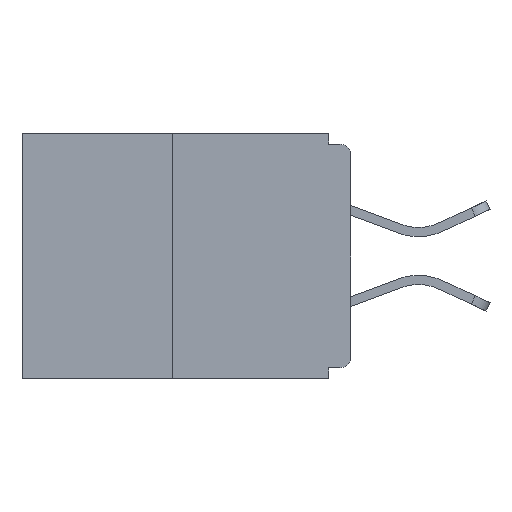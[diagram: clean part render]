
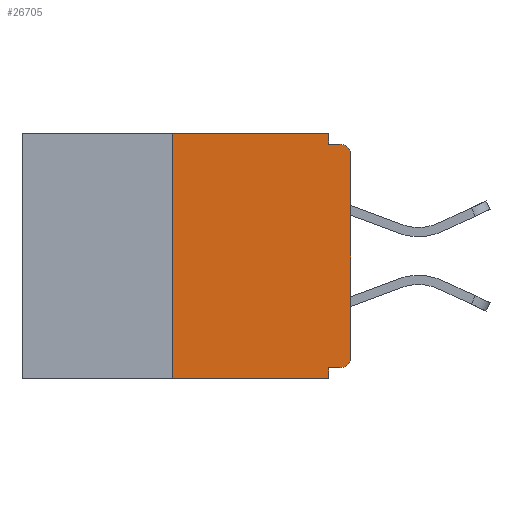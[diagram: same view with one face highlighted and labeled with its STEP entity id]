
A CAD part, left-side view. The second image highlights one B-rep face of the part: STEP entity #26705.
In plain terms, the highlighted planar face has unit normal (-1, 0, 0).
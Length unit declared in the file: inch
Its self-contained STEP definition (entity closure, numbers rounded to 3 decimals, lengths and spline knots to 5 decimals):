
#169 = VECTOR ( 'NONE', #17316, 39.37008 ) ;
#370 = ORIENTED_EDGE ( 'NONE', *, *, #10668, .T. ) ;
#379 = ORIENTED_EDGE ( 'NONE', *, *, #18137, .T. ) ;
#543 = DIRECTION ( 'NONE',  ( 0., 0., -1. ) ) ;
#657 = EDGE_LOOP ( 'NONE', ( #15188, #1661, #379, #4554, #2257, #5681, #370, #24033, #15216, #9652 ) ) ;
#1530 = DIRECTION ( 'NONE',  ( 0., 0., -1. ) ) ;
#1661 = ORIENTED_EDGE ( 'NONE', *, *, #25469, .F. ) ;
#1874 = VECTOR ( 'NONE', #26243, 39.37008 ) ;
#2257 = ORIENTED_EDGE ( 'NONE', *, *, #19185, .F. ) ;
#2644 = VECTOR ( 'NONE', #9814, 39.37008 ) ;
#2871 = VERTEX_POINT ( 'NONE', #27131 ) ;
#3639 = CARTESIAN_POINT ( 'NONE',  ( 0., 0.031, -0.328 ) ) ;
#3929 = VECTOR ( 'NONE', #16090, 39.37008 ) ;
#4485 = VERTEX_POINT ( 'NONE', #14809 ) ;
#4554 = ORIENTED_EDGE ( 'NONE', *, *, #28223, .F. ) ;
#4735 = DIRECTION ( 'NONE',  ( 0., 0., 1. ) ) ;
#5041 = EDGE_CURVE ( 'NONE', #23980, #18617, #19568, .T. ) ;
#5166 = AXIS2_PLACEMENT_3D ( 'NONE', #13131, #8432, #1530 ) ;
#5470 = LINE ( 'NONE', #19295, #26489 ) ;
#5681 = ORIENTED_EDGE ( 'NONE', *, *, #7123, .T. ) ;
#6280 = CARTESIAN_POINT ( 'NONE',  ( 0., 0.25, -0.343 ) ) ;
#7097 = CARTESIAN_POINT ( 'NONE',  ( 0., 0.25, 0. ) ) ;
#7123 = EDGE_CURVE ( 'NONE', #8736, #4485, #11064, .T. ) ;
#7246 = CARTESIAN_POINT ( 'NONE',  ( 0., 0.46, 0. ) ) ;
#7988 = LINE ( 'NONE', #18563, #3929 ) ;
#8432 = DIRECTION ( 'NONE',  ( -1., 0., 0. ) ) ;
#8517 = AXIS2_PLACEMENT_3D ( 'NONE', #17301, #24214, #19564 ) ;
#8670 = VERTEX_POINT ( 'NONE', #29027 ) ;
#8736 = VERTEX_POINT ( 'NONE', #10811 ) ;
#9028 = LINE ( 'NONE', #7097, #27049 ) ;
#9652 = ORIENTED_EDGE ( 'NONE', *, *, #22986, .F. ) ;
#9814 = DIRECTION ( 'NONE',  ( 0., -1., 0. ) ) ;
#10073 = VERTEX_POINT ( 'NONE', #18894 ) ;
#10401 = CARTESIAN_POINT ( 'NONE',  ( 0., 0., -0.328 ) ) ;
#10576 = DIRECTION ( 'NONE',  ( 0., 0., -1. ) ) ;
#10668 = EDGE_CURVE ( 'NONE', #4485, #8670, #15985, .T. ) ;
#10811 = CARTESIAN_POINT ( 'NONE',  ( 0., 0.015, -0.328 ) ) ;
#11064 = CIRCLE ( 'NONE', #8517, 0.015 ) ;
#11095 = LINE ( 'NONE', #23875, #1874 ) ;
#11470 = VERTEX_POINT ( 'NONE', #20252 ) ;
#13026 = DIRECTION ( 'NONE',  ( 0., 1., 0. ) ) ;
#13131 = CARTESIAN_POINT ( 'NONE',  ( 0., 0.015, -0.03 ) ) ;
#14470 = LINE ( 'NONE', #10401, #26305 ) ;
#14809 = CARTESIAN_POINT ( 'NONE',  ( 0., 0., -0.313 ) ) ;
#15131 = CARTESIAN_POINT ( 'NONE',  ( 0., 0., 0. ) ) ;
#15188 = ORIENTED_EDGE ( 'NONE', *, *, #27388, .F. ) ;
#15216 = ORIENTED_EDGE ( 'NONE', *, *, #5041, .F. ) ;
#15500 = FACE_OUTER_BOUND ( 'NONE', #657, .T. ) ;
#15985 = LINE ( 'NONE', #15131, #169 ) ;
#16090 = DIRECTION ( 'NONE',  ( 0., 0., -1. ) ) ;
#16686 = PLANE ( 'NONE',  #28862 ) ;
#17301 = CARTESIAN_POINT ( 'NONE',  ( 0., 0.015, -0.313 ) ) ;
#17316 = DIRECTION ( 'NONE',  ( 0., 0., 1. ) ) ;
#18137 = EDGE_CURVE ( 'NONE', #25332, #10073, #19724, .T. ) ;
#18244 = VECTOR ( 'NONE', #19646, 39.37008 ) ;
#18449 = VERTEX_POINT ( 'NONE', #3639 ) ;
#18563 = CARTESIAN_POINT ( 'NONE',  ( 0., 0.031, 0. ) ) ;
#18617 = VERTEX_POINT ( 'NONE', #22739 ) ;
#18894 = CARTESIAN_POINT ( 'NONE',  ( 0., 0.031, -0.343 ) ) ;
#19185 = EDGE_CURVE ( 'NONE', #8736, #18449, #14470, .T. ) ;
#19295 = CARTESIAN_POINT ( 'NONE',  ( 0., 0.031, -0.343 ) ) ;
#19564 = DIRECTION ( 'NONE',  ( 0., 0., -1. ) ) ;
#19568 = LINE ( 'NONE', #23787, #2644 ) ;
#19646 = DIRECTION ( 'NONE',  ( 0., -1., 0. ) ) ;
#19724 = LINE ( 'NONE', #19944, #18244 ) ;
#19944 = CARTESIAN_POINT ( 'NONE',  ( 0., 0.46, -0.343 ) ) ;
#20252 = CARTESIAN_POINT ( 'NONE',  ( 0., 0.25, 0. ) ) ;
#22212 = CIRCLE ( 'NONE', #5166, 0.015 ) ;
#22739 = CARTESIAN_POINT ( 'NONE',  ( 0., 0.015, -0.015 ) ) ;
#22986 = EDGE_CURVE ( 'NONE', #2871, #23980, #7988, .T. ) ;
#23787 = CARTESIAN_POINT ( 'NONE',  ( 0., 0., -0.015 ) ) ;
#23875 = CARTESIAN_POINT ( 'NONE',  ( 0., 0.46, 0. ) ) ;
#23980 = VERTEX_POINT ( 'NONE', #29234 ) ;
#24033 = ORIENTED_EDGE ( 'NONE', *, *, #25826, .T. ) ;
#24214 = DIRECTION ( 'NONE',  ( -1., 0., 0. ) ) ;
#25332 = VERTEX_POINT ( 'NONE', #6280 ) ;
#25469 = EDGE_CURVE ( 'NONE', #25332, #11470, #9028, .T. ) ;
#25826 = EDGE_CURVE ( 'NONE', #8670, #18617, #22212, .T. ) ;
#26243 = DIRECTION ( 'NONE',  ( 0., -1., 0. ) ) ;
#26305 = VECTOR ( 'NONE', #13026, 39.37008 ) ;
#26489 = VECTOR ( 'NONE', #10576, 39.37008 ) ;
#26705 = ADVANCED_FACE ( 'NONE', ( #15500 ), #16686, .F. ) ;
#27049 = VECTOR ( 'NONE', #4735, 39.37008 ) ;
#27131 = CARTESIAN_POINT ( 'NONE',  ( 0., 0.031, 0. ) ) ;
#27388 = EDGE_CURVE ( 'NONE', #11470, #2871, #11095, .T. ) ;
#28223 = EDGE_CURVE ( 'NONE', #18449, #10073, #5470, .T. ) ;
#28568 = DIRECTION ( 'NONE',  ( 1., 0., 0. ) ) ;
#28862 = AXIS2_PLACEMENT_3D ( 'NONE', #7246, #28568, #543 ) ;
#29027 = CARTESIAN_POINT ( 'NONE',  ( 0., 0., -0.03 ) ) ;
#29234 = CARTESIAN_POINT ( 'NONE',  ( 0., 0.031, -0.015 ) ) ;
